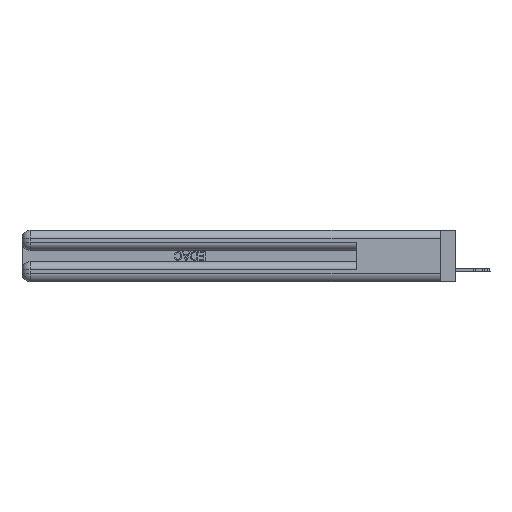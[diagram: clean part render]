
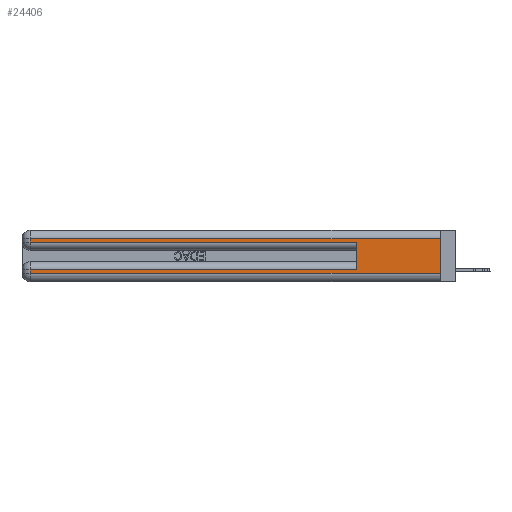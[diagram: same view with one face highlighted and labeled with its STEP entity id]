
A CAD part, left-side view. The second image highlights one B-rep face of the part: STEP entity #24406.
In plain terms, the highlighted planar face has unit normal (-1, 0, 0).
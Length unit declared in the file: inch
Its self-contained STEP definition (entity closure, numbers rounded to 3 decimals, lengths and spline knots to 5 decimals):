
#1369 = CARTESIAN_POINT ( 'NONE',  ( 0., 2.94, 0.06 ) ) ;
#2026 = CARTESIAN_POINT ( 'NONE',  ( 0., 0., 0.06 ) ) ;
#2388 = ORIENTED_EDGE ( 'NONE', *, *, #44749, .F. ) ;
#2449 = DIRECTION ( 'NONE',  ( 0., 0., -1. ) ) ;
#3019 = VECTOR ( 'NONE', #12228, 39.37008 ) ;
#3307 = CARTESIAN_POINT ( 'NONE',  ( 0., 0., 0.37 ) ) ;
#3507 = ORIENTED_EDGE ( 'NONE', *, *, #18001, .T. ) ;
#3749 = VECTOR ( 'NONE', #39878, 39.37008 ) ;
#4732 = CARTESIAN_POINT ( 'NONE',  ( 0., 0., 0.31 ) ) ;
#5074 = EDGE_CURVE ( 'NONE', #13664, #35485, #30943, .T. ) ;
#8675 = EDGE_CURVE ( 'NONE', #18721, #35485, #39731, .T. ) ;
#9150 = CARTESIAN_POINT ( 'NONE',  ( 0., 2.94, 0.37 ) ) ;
#9203 = VECTOR ( 'NONE', #31571, 39.37008 ) ;
#9332 = LINE ( 'NONE', #9150, #3019 ) ;
#9351 = EDGE_CURVE ( 'NONE', #29412, #29941, #20932, .T. ) ;
#11015 = EDGE_CURVE ( 'NONE', #29941, #18721, #9332, .T. ) ;
#11957 = DIRECTION ( 'NONE',  ( 0., 1., 0. ) ) ;
#12017 = CARTESIAN_POINT ( 'NONE',  ( 0., 0., 0.06 ) ) ;
#12228 = DIRECTION ( 'NONE',  ( 0., 0., -1. ) ) ;
#13621 = LINE ( 'NONE', #13677, #40938 ) ;
#13664 = VERTEX_POINT ( 'NONE', #36710 ) ;
#13677 = CARTESIAN_POINT ( 'NONE',  ( 0., 2.94, 0.37 ) ) ;
#14651 = VECTOR ( 'NONE', #33239, 39.37008 ) ;
#14738 = EDGE_CURVE ( 'NONE', #23488, #19240, #13621, .T. ) ;
#16934 = VECTOR ( 'NONE', #11957, 39.37008 ) ;
#17060 = CARTESIAN_POINT ( 'NONE',  ( 0., 0.6, 0.145 ) ) ;
#17689 = ORIENTED_EDGE ( 'NONE', *, *, #5074, .F. ) ;
#18001 = EDGE_CURVE ( 'NONE', #19240, #44238, #38314, .T. ) ;
#18721 = VERTEX_POINT ( 'NONE', #31662 ) ;
#19240 = VERTEX_POINT ( 'NONE', #1369 ) ;
#19399 = CARTESIAN_POINT ( 'NONE',  ( 0., 2.94, 0.31 ) ) ;
#19750 = ORIENTED_EDGE ( 'NONE', *, *, #14738, .T. ) ;
#20907 = DIRECTION ( 'NONE',  ( 0., 0., 1. ) ) ;
#20932 = LINE ( 'NONE', #33330, #16934 ) ;
#22534 = EDGE_LOOP ( 'NONE', ( #2388, #44888, #42655, #41609, #17689, #30124, #19750, #3507 ) ) ;
#23102 = EDGE_CURVE ( 'NONE', #13664, #23488, #29497, .T. ) ;
#23488 = VERTEX_POINT ( 'NONE', #35222 ) ;
#23746 = AXIS2_PLACEMENT_3D ( 'NONE', #28808, #40563, #33087 ) ;
#24216 = FACE_OUTER_BOUND ( 'NONE', #22534, .T. ) ;
#24406 = ADVANCED_FACE ( 'NONE', ( #24216 ), #32923, .F. ) ;
#27617 = CARTESIAN_POINT ( 'NONE',  ( 0., 0.6, 0.285 ) ) ;
#28808 = CARTESIAN_POINT ( 'NONE',  ( 0., 0., 0.37 ) ) ;
#29412 = VERTEX_POINT ( 'NONE', #4732 ) ;
#29497 = LINE ( 'NONE', #36232, #3749 ) ;
#29941 = VERTEX_POINT ( 'NONE', #19399 ) ;
#30124 = ORIENTED_EDGE ( 'NONE', *, *, #23102, .T. ) ;
#30943 = LINE ( 'NONE', #17060, #36062 ) ;
#31571 = DIRECTION ( 'NONE',  ( 0., -1., 0. ) ) ;
#31662 = CARTESIAN_POINT ( 'NONE',  ( 0., 2.94, 0.285 ) ) ;
#32923 = PLANE ( 'NONE',  #23746 ) ;
#33087 = DIRECTION ( 'NONE',  ( 0., 0., -1. ) ) ;
#33239 = DIRECTION ( 'NONE',  ( 0., -1., 0. ) ) ;
#33330 = CARTESIAN_POINT ( 'NONE',  ( 0., 0., 0.31 ) ) ;
#33472 = DIRECTION ( 'NONE',  ( 0., 0., -1. ) ) ;
#33530 = CARTESIAN_POINT ( 'NONE',  ( 0., 0., 0.285 ) ) ;
#35222 = CARTESIAN_POINT ( 'NONE',  ( 0., 2.94, 0.085 ) ) ;
#35485 = VERTEX_POINT ( 'NONE', #27617 ) ;
#36062 = VECTOR ( 'NONE', #20907, 39.37008 ) ;
#36232 = CARTESIAN_POINT ( 'NONE',  ( 0., 0., 0.085 ) ) ;
#36710 = CARTESIAN_POINT ( 'NONE',  ( 0., 0.6, 0.085 ) ) ;
#38314 = LINE ( 'NONE', #2026, #9203 ) ;
#39452 = VECTOR ( 'NONE', #33472, 39.37008 ) ;
#39731 = LINE ( 'NONE', #33530, #14651 ) ;
#39878 = DIRECTION ( 'NONE',  ( 0., 1., 0. ) ) ;
#40563 = DIRECTION ( 'NONE',  ( 1., 0., 0. ) ) ;
#40595 = LINE ( 'NONE', #3307, #39452 ) ;
#40938 = VECTOR ( 'NONE', #2449, 39.37008 ) ;
#41609 = ORIENTED_EDGE ( 'NONE', *, *, #8675, .T. ) ;
#42655 = ORIENTED_EDGE ( 'NONE', *, *, #11015, .T. ) ;
#44238 = VERTEX_POINT ( 'NONE', #12017 ) ;
#44749 = EDGE_CURVE ( 'NONE', #29412, #44238, #40595, .T. ) ;
#44888 = ORIENTED_EDGE ( 'NONE', *, *, #9351, .T. ) ;
